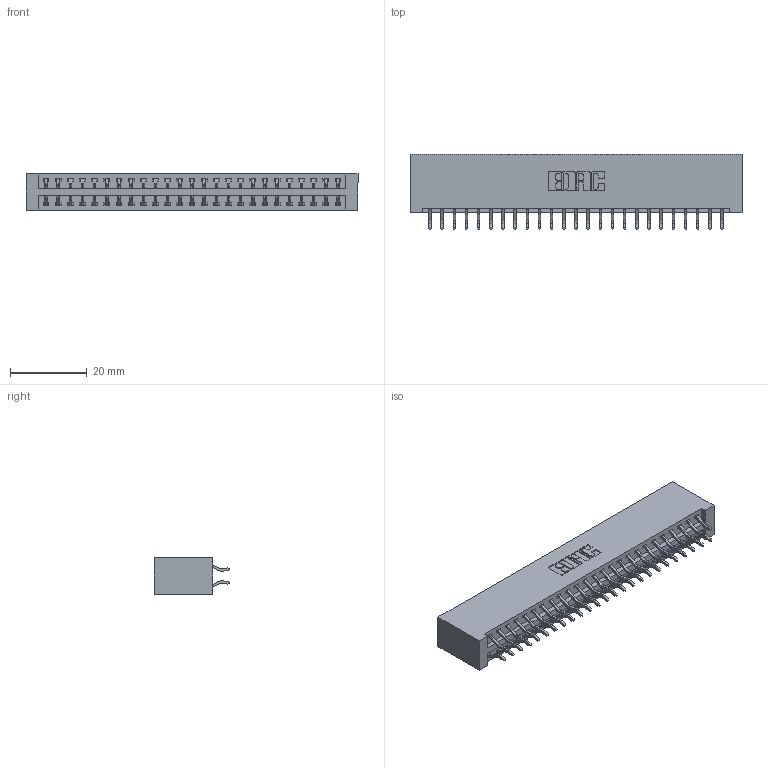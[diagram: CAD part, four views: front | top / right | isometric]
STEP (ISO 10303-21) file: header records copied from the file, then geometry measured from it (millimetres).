
FILE_DESCRIPTION (( 'STEP AP203' ), '1' );
FILE_NAME ('396-050-556-201.STEP', '2019-10-30T13:15:20', ( '' ), ( '' ), 'SwSTEP 2.0', 'SolidWorks 2016', '' );
FILE_SCHEMA (( 'CONFIG_CONTROL_DESIGN' ));
Length unit declared in the file: inch
Products named in the file (3): 396-050-556-201; 345-292-001_556 Tail; 346 Part_No Mounting Lugs
Assembly tree (51 placements, depth 2):
  396-050-556-201
    346 Part_No Mounting Lugs
    345-292-001_556 Tail  x50
Bounding box: 86.61 x 19.57 x 9.4 mm (x, y, z)
Volume: 8885.2 mm3; surface area: 12062.9 mm2
Topology: 51 solids, 51 shells, 3014 faces, 8955 edges, 5902 vertices
Faces by surface type: plane 2022, cylinder 992
Entity records: 18547 total; most frequent: CARTESIAN_POINT 3092, ORIENTED_EDGE 3014, DIRECTION 2759, EDGE_CURVE 1507, LINE 1275, VECTOR 1275, VERTEX_POINT 1002, AXIS2_PLACEMENT_3D 742
